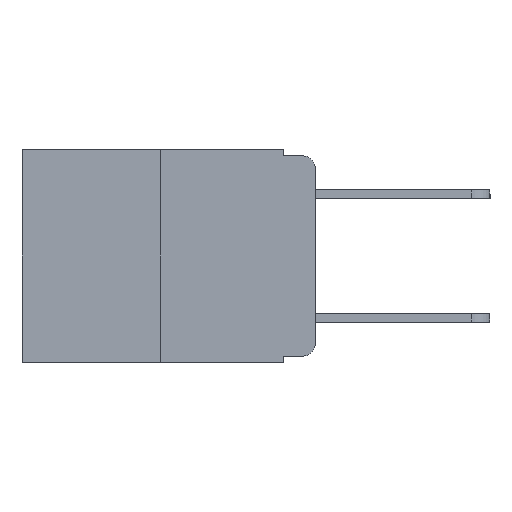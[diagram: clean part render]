
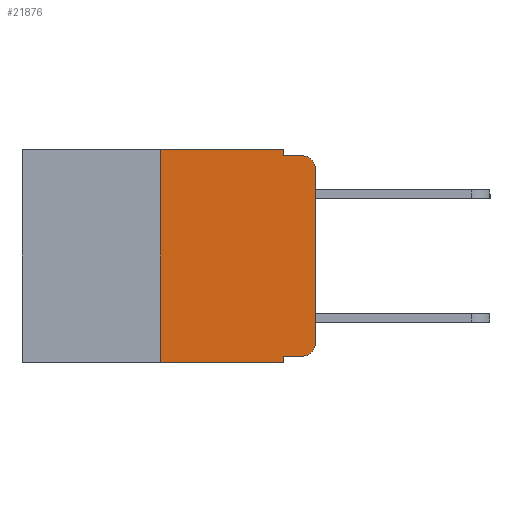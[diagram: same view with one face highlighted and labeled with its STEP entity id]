
A CAD part, left-side view. The second image highlights one B-rep face of the part: STEP entity #21876.
In plain terms, the highlighted planar face has unit normal (-1, 0, 0).
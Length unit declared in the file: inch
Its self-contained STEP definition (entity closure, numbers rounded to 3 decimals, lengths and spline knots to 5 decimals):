
#52 = DIRECTION ( 'NONE',  ( 0., 0., -1. ) ) ;
#135 = DIRECTION ( 'NONE',  ( 0., 0., -1. ) ) ;
#242 = VECTOR ( 'NONE', #18322, 39.37008 ) ;
#532 = DIRECTION ( 'NONE',  ( 0., -1., 0. ) ) ;
#1409 = CARTESIAN_POINT ( 'NONE',  ( 0., 0.02, -0.313 ) ) ;
#1558 = CIRCLE ( 'NONE', #11546, 0.02 ) ;
#1695 = CARTESIAN_POINT ( 'NONE',  ( 0., 0.25, 0. ) ) ;
#1723 = DIRECTION ( 'NONE',  ( 0., 0., -1. ) ) ;
#1825 = LINE ( 'NONE', #12730, #12349 ) ;
#1851 = VECTOR ( 'NONE', #1723, 39.37008 ) ;
#1891 = CARTESIAN_POINT ( 'NONE',  ( 0., 0.02, -0.333 ) ) ;
#2593 = CARTESIAN_POINT ( 'NONE',  ( 0., 0.051, -0.01 ) ) ;
#3155 = DIRECTION ( 'NONE',  ( 0., -1., 0. ) ) ;
#3307 = VECTOR ( 'NONE', #3155, 39.37008 ) ;
#3316 = DIRECTION ( 'NONE',  ( 0., 0., 1. ) ) ;
#3378 = VERTEX_POINT ( 'NONE', #5525 ) ;
#3538 = CARTESIAN_POINT ( 'NONE',  ( 0., 0.25, 0. ) ) ;
#3558 = DIRECTION ( 'NONE',  ( 0., 0., -1. ) ) ;
#3964 = EDGE_CURVE ( 'NONE', #3378, #23212, #14384, .T. ) ;
#4071 = ORIENTED_EDGE ( 'NONE', *, *, #14939, .T. ) ;
#4261 = PLANE ( 'NONE',  #18237 ) ;
#4455 = CIRCLE ( 'NONE', #17747, 0.02 ) ;
#4877 = EDGE_CURVE ( 'NONE', #19547, #5968, #5930, .T. ) ;
#5525 = CARTESIAN_POINT ( 'NONE',  ( 0., 0.051, -0.333 ) ) ;
#5837 = VERTEX_POINT ( 'NONE', #23597 ) ;
#5930 = LINE ( 'NONE', #1695, #242 ) ;
#5968 = VERTEX_POINT ( 'NONE', #3538 ) ;
#6648 = EDGE_CURVE ( 'NONE', #18552, #12921, #24333, .T. ) ;
#7153 = LINE ( 'NONE', #24293, #18083 ) ;
#7165 = EDGE_CURVE ( 'NONE', #5837, #18552, #1825, .T. ) ;
#7494 = LINE ( 'NONE', #10119, #1851 ) ;
#7635 = CARTESIAN_POINT ( 'NONE',  ( 0., 0.02, -0.01 ) ) ;
#7675 = ORIENTED_EDGE ( 'NONE', *, *, #12374, .F. ) ;
#8082 = DIRECTION ( 'NONE',  ( 0., -1., 0. ) ) ;
#10119 = CARTESIAN_POINT ( 'NONE',  ( 0., 0.051, 0. ) ) ;
#11058 = LINE ( 'NONE', #17797, #25867 ) ;
#11546 = AXIS2_PLACEMENT_3D ( 'NONE', #1409, #15991, #3558 ) ;
#11731 = DIRECTION ( 'NONE',  ( -1., 0., 0. ) ) ;
#12349 = VECTOR ( 'NONE', #135, 39.37008 ) ;
#12374 = EDGE_CURVE ( 'NONE', #3378, #12608, #7494, .T. ) ;
#12547 = EDGE_CURVE ( 'NONE', #5968, #5837, #19355, .T. ) ;
#12608 = VERTEX_POINT ( 'NONE', #18953 ) ;
#12618 = ORIENTED_EDGE ( 'NONE', *, *, #6648, .F. ) ;
#12656 = DIRECTION ( 'NONE',  ( 1., 0., 0. ) ) ;
#12730 = CARTESIAN_POINT ( 'NONE',  ( 0., 0.051, 0. ) ) ;
#12921 = VERTEX_POINT ( 'NONE', #7635 ) ;
#13865 = ORIENTED_EDGE ( 'NONE', *, *, #21016, .T. ) ;
#13885 = EDGE_CURVE ( 'NONE', #19547, #12608, #7153, .T. ) ;
#14384 = LINE ( 'NONE', #25584, #3307 ) ;
#14906 = ORIENTED_EDGE ( 'NONE', *, *, #4877, .F. ) ;
#14939 = EDGE_CURVE ( 'NONE', #20928, #12921, #4455, .T. ) ;
#15564 = CARTESIAN_POINT ( 'NONE',  ( 0., 0., -0.313 ) ) ;
#15991 = DIRECTION ( 'NONE',  ( -1., 0., 0. ) ) ;
#17203 = EDGE_LOOP ( 'NONE', ( #21094, #4071, #12618, #18677, #17767, #14906, #18542, #7675, #22340, #13865 ) ) ;
#17603 = VERTEX_POINT ( 'NONE', #15564 ) ;
#17688 = CARTESIAN_POINT ( 'NONE',  ( 0., 0., -0.03 ) ) ;
#17747 = AXIS2_PLACEMENT_3D ( 'NONE', #23810, #11731, #25820 ) ;
#17767 = ORIENTED_EDGE ( 'NONE', *, *, #12547, .F. ) ;
#17797 = CARTESIAN_POINT ( 'NONE',  ( 0., 0., 0. ) ) ;
#18083 = VECTOR ( 'NONE', #8082, 39.37008 ) ;
#18237 = AXIS2_PLACEMENT_3D ( 'NONE', #18699, #12656, #52 ) ;
#18322 = DIRECTION ( 'NONE',  ( 0., 0., 1. ) ) ;
#18542 = ORIENTED_EDGE ( 'NONE', *, *, #13885, .T. ) ;
#18552 = VERTEX_POINT ( 'NONE', #22724 ) ;
#18677 = ORIENTED_EDGE ( 'NONE', *, *, #7165, .F. ) ;
#18699 = CARTESIAN_POINT ( 'NONE',  ( 0., 0.473, 0. ) ) ;
#18953 = CARTESIAN_POINT ( 'NONE',  ( 0., 0.051, -0.343 ) ) ;
#19056 = VECTOR ( 'NONE', #532, 39.37008 ) ;
#19355 = LINE ( 'NONE', #20783, #19976 ) ;
#19547 = VERTEX_POINT ( 'NONE', #24899 ) ;
#19976 = VECTOR ( 'NONE', #22697, 39.37008 ) ;
#20783 = CARTESIAN_POINT ( 'NONE',  ( 0., 0.473, 0. ) ) ;
#20928 = VERTEX_POINT ( 'NONE', #17688 ) ;
#21016 = EDGE_CURVE ( 'NONE', #23212, #17603, #1558, .T. ) ;
#21094 = ORIENTED_EDGE ( 'NONE', *, *, #22199, .T. ) ;
#21876 = ADVANCED_FACE ( 'NONE', ( #23390 ), #4261, .F. ) ;
#22199 = EDGE_CURVE ( 'NONE', #17603, #20928, #11058, .T. ) ;
#22340 = ORIENTED_EDGE ( 'NONE', *, *, #3964, .T. ) ;
#22697 = DIRECTION ( 'NONE',  ( 0., -1., 0. ) ) ;
#22724 = CARTESIAN_POINT ( 'NONE',  ( 0., 0.051, -0.01 ) ) ;
#23212 = VERTEX_POINT ( 'NONE', #1891 ) ;
#23390 = FACE_OUTER_BOUND ( 'NONE', #17203, .T. ) ;
#23597 = CARTESIAN_POINT ( 'NONE',  ( 0., 0.051, 0. ) ) ;
#23810 = CARTESIAN_POINT ( 'NONE',  ( 0., 0.02, -0.03 ) ) ;
#24293 = CARTESIAN_POINT ( 'NONE',  ( 0., 0.473, -0.343 ) ) ;
#24333 = LINE ( 'NONE', #2593, #19056 ) ;
#24899 = CARTESIAN_POINT ( 'NONE',  ( 0., 0.25, -0.343 ) ) ;
#25584 = CARTESIAN_POINT ( 'NONE',  ( 0., 0.051, -0.333 ) ) ;
#25820 = DIRECTION ( 'NONE',  ( 0., 0., -1. ) ) ;
#25867 = VECTOR ( 'NONE', #3316, 39.37008 ) ;
